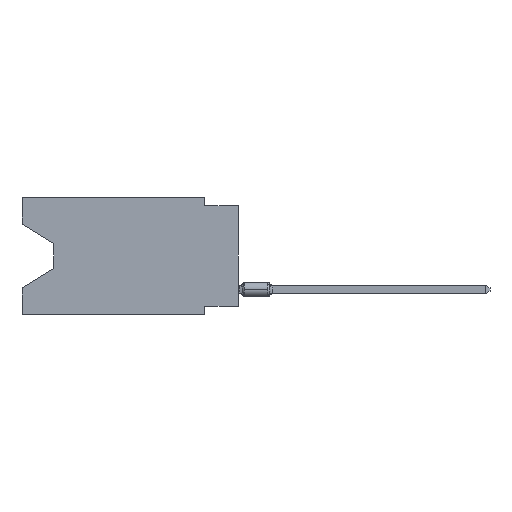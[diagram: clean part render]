
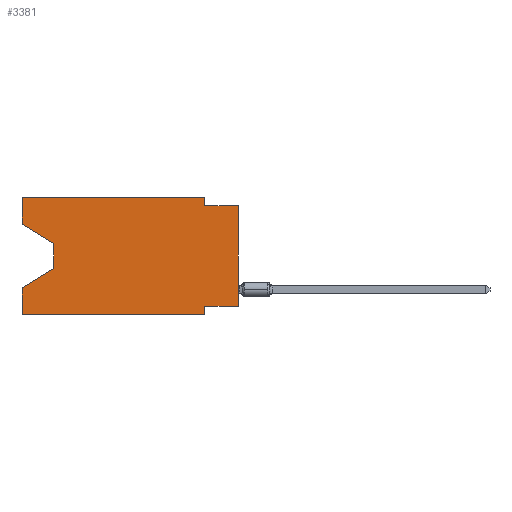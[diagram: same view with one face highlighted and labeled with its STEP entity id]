
A CAD part, left-side view. The second image highlights one B-rep face of the part: STEP entity #3381.
In plain terms, the highlighted planar face has unit normal (-1, 0, 0).
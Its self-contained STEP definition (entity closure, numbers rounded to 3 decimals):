
#118 = FACE_OUTER_BOUND ( 'NONE', #6412, .T. ) ;
#227 = CARTESIAN_POINT ( 'NONE',  ( 0., 2.54, 0. ) ) ;
#1632 = DIRECTION ( 'NONE',  ( 0., 0.855, -0.519 ) ) ;
#2356 = LINE ( 'NONE', #15259, #22367 ) ;
#3113 = CARTESIAN_POINT ( 'NONE',  ( 0., 16.383, 0. ) ) ;
#3185 = ORIENTED_EDGE ( 'NONE', *, *, #25718, .T. ) ;
#3381 = ADVANCED_FACE ( 'NONE', ( #118 ), #13299, .F. ) ;
#3536 = LINE ( 'NONE', #28281, #5432 ) ;
#4495 = ORIENTED_EDGE ( 'NONE', *, *, #25425, .F. ) ;
#4506 = VECTOR ( 'NONE', #15213, 1000. ) ;
#4877 = CARTESIAN_POINT ( 'NONE',  ( 0., 0., -0.635 ) ) ;
#5432 = VECTOR ( 'NONE', #1632, 1000. ) ;
#5637 = LINE ( 'NONE', #12359, #17115 ) ;
#5866 = AXIS2_PLACEMENT_3D ( 'NONE', #28967, #8909, #24730 ) ;
#5981 = VECTOR ( 'NONE', #21122, 1000. ) ;
#6037 = EDGE_CURVE ( 'NONE', #10334, #9480, #16321, .T. ) ;
#6412 = EDGE_LOOP ( 'NONE', ( #12192, #24753, #3185, #18868, #17009, #4495, #24915, #13922, #27326, #26752, #21461, #23096 ) ) ;
#7052 = CARTESIAN_POINT ( 'NONE',  ( 0., 2.54, -0.635 ) ) ;
#7592 = VERTEX_POINT ( 'NONE', #8969 ) ;
#7707 = VERTEX_POINT ( 'NONE', #18051 ) ;
#8286 = VERTEX_POINT ( 'NONE', #7052 ) ;
#8725 = CARTESIAN_POINT ( 'NONE',  ( 0., 13.97, -5.385 ) ) ;
#8909 = DIRECTION ( 'NONE',  ( 1., 0., 0. ) ) ;
#8969 = CARTESIAN_POINT ( 'NONE',  ( 0., 16.383, 0. ) ) ;
#9223 = VECTOR ( 'NONE', #12054, 1000. ) ;
#9444 = CARTESIAN_POINT ( 'NONE',  ( 0., 16.383, -6.852 ) ) ;
#9480 = VERTEX_POINT ( 'NONE', #13819 ) ;
#9863 = VERTEX_POINT ( 'NONE', #23289 ) ;
#9935 = LINE ( 'NONE', #22976, #24850 ) ;
#10210 = CARTESIAN_POINT ( 'NONE',  ( 0., 13.97, -3.505 ) ) ;
#10212 = VECTOR ( 'NONE', #21154, 1000. ) ;
#10334 = VERTEX_POINT ( 'NONE', #26161 ) ;
#10512 = VERTEX_POINT ( 'NONE', #8725 ) ;
#10538 = EDGE_CURVE ( 'NONE', #10334, #7707, #10921, .T. ) ;
#10921 = LINE ( 'NONE', #17945, #16424 ) ;
#12054 = DIRECTION ( 'NONE',  ( 0., 0., 1. ) ) ;
#12192 = ORIENTED_EDGE ( 'NONE', *, *, #28556, .T. ) ;
#12216 = LINE ( 'NONE', #14412, #10212 ) ;
#12359 = CARTESIAN_POINT ( 'NONE',  ( 0., 2.54, -8.89 ) ) ;
#12906 = VECTOR ( 'NONE', #18944, 1000. ) ;
#13299 = PLANE ( 'NONE',  #5866 ) ;
#13497 = VERTEX_POINT ( 'NONE', #10210 ) ;
#13819 = CARTESIAN_POINT ( 'NONE',  ( 0., 2.54, -8.255 ) ) ;
#13922 = ORIENTED_EDGE ( 'NONE', *, *, #10538, .T. ) ;
#14109 = DIRECTION ( 'NONE',  ( 0., 1., 0. ) ) ;
#14412 = CARTESIAN_POINT ( 'NONE',  ( 0., 16.383, -8.89 ) ) ;
#15213 = DIRECTION ( 'NONE',  ( 0., 0., 1. ) ) ;
#15259 = CARTESIAN_POINT ( 'NONE',  ( 0., 13.97, -3.505 ) ) ;
#15882 = CARTESIAN_POINT ( 'NONE',  ( 0., 0., -8.255 ) ) ;
#16111 = VERTEX_POINT ( 'NONE', #21202 ) ;
#16321 = LINE ( 'NONE', #15882, #22299 ) ;
#16400 = VERTEX_POINT ( 'NONE', #227 ) ;
#16424 = VECTOR ( 'NONE', #20017, 1000. ) ;
#16854 = EDGE_CURVE ( 'NONE', #8286, #7707, #23335, .T. ) ;
#16983 = LINE ( 'NONE', #28534, #4506 ) ;
#17009 = ORIENTED_EDGE ( 'NONE', *, *, #19135, .T. ) ;
#17086 = EDGE_CURVE ( 'NONE', #13497, #10512, #2356, .T. ) ;
#17087 = CARTESIAN_POINT ( 'NONE',  ( 0., 16.383, 0. ) ) ;
#17115 = VECTOR ( 'NONE', #21303, 1000. ) ;
#17186 = CARTESIAN_POINT ( 'NONE',  ( 0., 2.54, 0. ) ) ;
#17453 = DIRECTION ( 'NONE',  ( 0., 0., -1. ) ) ;
#17945 = CARTESIAN_POINT ( 'NONE',  ( 0., 0., 0. ) ) ;
#18051 = CARTESIAN_POINT ( 'NONE',  ( 0., 0., -0.635 ) ) ;
#18178 = EDGE_CURVE ( 'NONE', #21722, #7592, #23197, .T. ) ;
#18868 = ORIENTED_EDGE ( 'NONE', *, *, #24497, .F. ) ;
#18944 = DIRECTION ( 'NONE',  ( 0., 0., -1. ) ) ;
#19135 = EDGE_CURVE ( 'NONE', #9863, #16111, #12216, .T. ) ;
#19976 = EDGE_CURVE ( 'NONE', #16400, #8286, #26124, .T. ) ;
#20017 = DIRECTION ( 'NONE',  ( 0., 0., 1. ) ) ;
#21122 = DIRECTION ( 'NONE',  ( 0., -1., 0. ) ) ;
#21154 = DIRECTION ( 'NONE',  ( 0., -1., 0. ) ) ;
#21202 = CARTESIAN_POINT ( 'NONE',  ( 0., 2.54, -8.89 ) ) ;
#21212 = DIRECTION ( 'NONE',  ( 0., -0.855, -0.519 ) ) ;
#21303 = DIRECTION ( 'NONE',  ( 0., 0., -1. ) ) ;
#21461 = ORIENTED_EDGE ( 'NONE', *, *, #22464, .F. ) ;
#21722 = VERTEX_POINT ( 'NONE', #24190 ) ;
#22299 = VECTOR ( 'NONE', #14109, 1000. ) ;
#22367 = VECTOR ( 'NONE', #17453, 1000. ) ;
#22464 = EDGE_CURVE ( 'NONE', #7592, #16400, #23830, .T. ) ;
#22976 = CARTESIAN_POINT ( 'NONE',  ( 0., 16.383, -2.038 ) ) ;
#23096 = ORIENTED_EDGE ( 'NONE', *, *, #18178, .F. ) ;
#23197 = LINE ( 'NONE', #3113, #9223 ) ;
#23289 = CARTESIAN_POINT ( 'NONE',  ( 0., 16.383, -8.89 ) ) ;
#23335 = LINE ( 'NONE', #4877, #5981 ) ;
#23830 = LINE ( 'NONE', #17087, #25042 ) ;
#24190 = CARTESIAN_POINT ( 'NONE',  ( 0., 16.383, -2.038 ) ) ;
#24497 = EDGE_CURVE ( 'NONE', #9863, #25258, #16983, .T. ) ;
#24730 = DIRECTION ( 'NONE',  ( 0., 0., -1. ) ) ;
#24753 = ORIENTED_EDGE ( 'NONE', *, *, #17086, .T. ) ;
#24850 = VECTOR ( 'NONE', #21212, 1000. ) ;
#24915 = ORIENTED_EDGE ( 'NONE', *, *, #6037, .F. ) ;
#25042 = VECTOR ( 'NONE', #28497, 1000. ) ;
#25258 = VERTEX_POINT ( 'NONE', #9444 ) ;
#25425 = EDGE_CURVE ( 'NONE', #9480, #16111, #5637, .T. ) ;
#25718 = EDGE_CURVE ( 'NONE', #10512, #25258, #3536, .T. ) ;
#26124 = LINE ( 'NONE', #17186, #12906 ) ;
#26161 = CARTESIAN_POINT ( 'NONE',  ( 0., 0., -8.255 ) ) ;
#26752 = ORIENTED_EDGE ( 'NONE', *, *, #19976, .F. ) ;
#27326 = ORIENTED_EDGE ( 'NONE', *, *, #16854, .F. ) ;
#28281 = CARTESIAN_POINT ( 'NONE',  ( 0., 13.97, -5.385 ) ) ;
#28497 = DIRECTION ( 'NONE',  ( 0., -1., 0. ) ) ;
#28534 = CARTESIAN_POINT ( 'NONE',  ( 0., 16.383, 0. ) ) ;
#28556 = EDGE_CURVE ( 'NONE', #21722, #13497, #9935, .T. ) ;
#28967 = CARTESIAN_POINT ( 'NONE',  ( 0., 16.383, 0. ) ) ;
